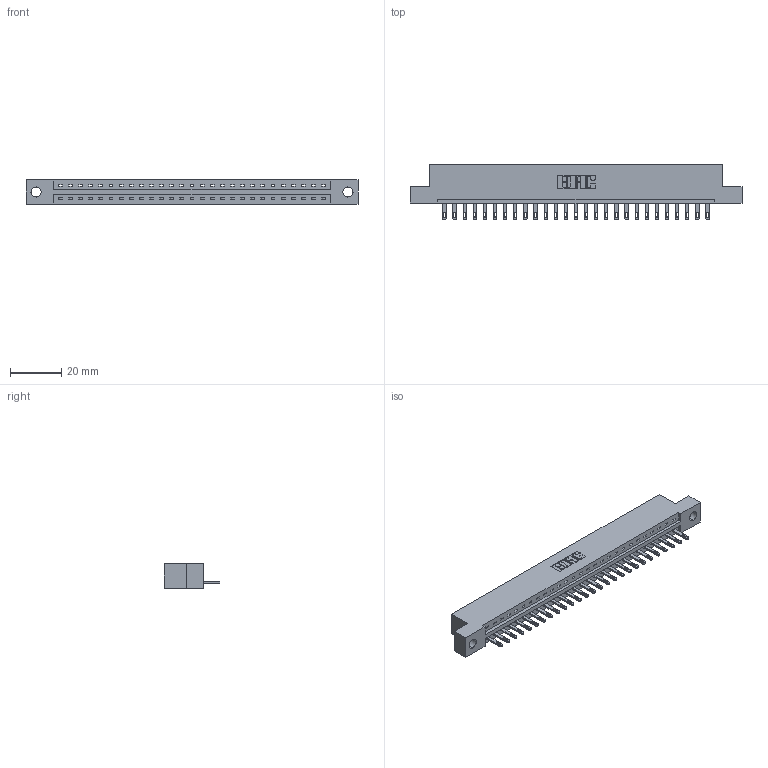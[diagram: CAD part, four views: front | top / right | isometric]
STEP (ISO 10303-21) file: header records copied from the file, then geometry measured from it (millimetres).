
FILE_DESCRIPTION (( 'STEP AP203' ), '1' );
FILE_NAME ('337-027-500-104.STEP', '2018-08-06T07:04:08', ( '' ), ( '' ), 'SwSTEP 2.0', 'SolidWorks 2016', '' );
FILE_SCHEMA (( 'CONFIG_CONTROL_DESIGN' ));
Length unit declared in the file: inch
Products named in the file (3): 337 Part_Flush Mounting Lugs - 0.156 Dia-TH; 345-292-001_345-293-100; 337-027-500-104
Assembly tree (28 placements, depth 2):
  337-027-500-104
    337 Part_Flush Mounting Lugs - 0.156 Dia-TH
    345-292-001_345-293-100  x27
Bounding box: 130 x 21.85 x 9.4 mm (x, y, z)
Volume: 13252.2 mm3; surface area: 13469.2 mm2
Topology: 28 solids, 28 shells, 1680 faces, 5171 edges, 3446 vertices
Faces by surface type: plane 1150, cylinder 530
Entity records: 21943 total; most frequent: CARTESIAN_POINT 3827, ORIENTED_EDGE 3790, DIRECTION 3253, EDGE_CURVE 1895, VECTOR 1763, LINE 1763, VERTEX_POINT 1262, AXIS2_PLACEMENT_3D 745
